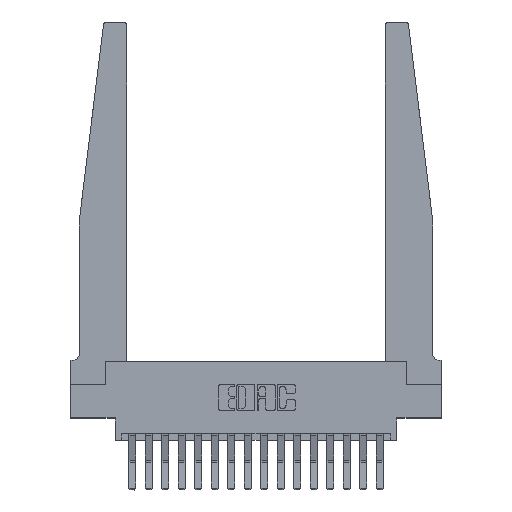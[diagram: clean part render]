
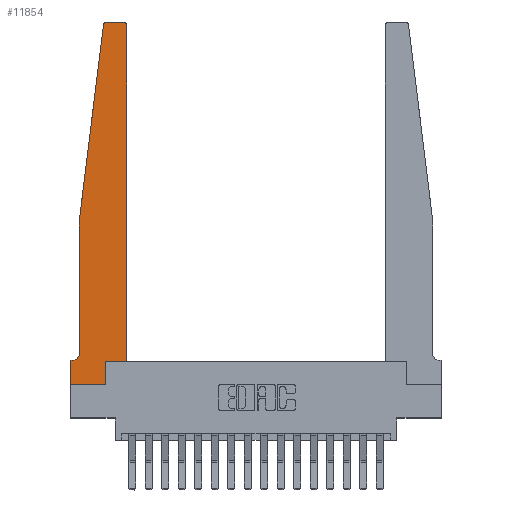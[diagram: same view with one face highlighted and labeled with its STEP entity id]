
A CAD part, top view. The second image highlights one B-rep face of the part: STEP entity #11854.
In plain terms, the highlighted planar face has unit normal (0, 0, 1).
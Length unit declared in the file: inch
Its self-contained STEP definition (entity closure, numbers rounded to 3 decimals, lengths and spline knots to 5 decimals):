
#161 = LINE ( 'NONE', #13984, #15330 ) ;
#328 = DIRECTION ( 'NONE',  ( 1., 0., 0. ) ) ;
#408 = LINE ( 'NONE', #9254, #11677 ) ;
#550 = EDGE_CURVE ( 'NONE', #15427, #4599, #3667, .T. ) ;
#650 = VERTEX_POINT ( 'NONE', #6607 ) ;
#772 = EDGE_CURVE ( 'NONE', #4599, #8223, #408, .T. ) ;
#826 = CARTESIAN_POINT ( 'NONE',  ( 0., 0., 0.37 ) ) ;
#884 = LINE ( 'NONE', #16039, #11665 ) ;
#1208 = DIRECTION ( 'NONE',  ( -1., 0., 0. ) ) ;
#1330 = EDGE_CURVE ( 'NONE', #14689, #12836, #15918, .T. ) ;
#1644 = CARTESIAN_POINT ( 'NONE',  ( 0.2605, 0.18, 0.37 ) ) ;
#1951 = CARTESIAN_POINT ( 'NONE',  ( 0.425, 0.18, 0.37 ) ) ;
#2693 = DIRECTION ( 'NONE',  ( 1., 0., 0. ) ) ;
#2923 = LINE ( 'NONE', #10007, #7752 ) ;
#3080 = EDGE_CURVE ( 'NONE', #8223, #14689, #9903, .T. ) ;
#3102 = ORIENTED_EDGE ( 'NONE', *, *, #15533, .T. ) ;
#3667 = LINE ( 'NONE', #1644, #18259 ) ;
#4114 = CARTESIAN_POINT ( 'NONE',  ( 0.065, 1.25, 0.37 ) ) ;
#4512 = CARTESIAN_POINT ( 'NONE',  ( 0.065, 1.25, 0.37 ) ) ;
#4599 = VERTEX_POINT ( 'NONE', #17142 ) ;
#4915 = CARTESIAN_POINT ( 'NONE',  ( 0.24675, 2.72367, 0.37 ) ) ;
#4948 = ORIENTED_EDGE ( 'NONE', *, *, #772, .T. ) ;
#5209 = LINE ( 'NONE', #4114, #16423 ) ;
#5229 = VERTEX_POINT ( 'NONE', #6952 ) ;
#5398 = DIRECTION ( 'NONE',  ( 1., 0., 0. ) ) ;
#5620 = AXIS2_PLACEMENT_3D ( 'NONE', #13778, #14195, #5398 ) ;
#6065 = VERTEX_POINT ( 'NONE', #4915 ) ;
#6173 = CARTESIAN_POINT ( 'NONE',  ( 0., 0.1875, 0.37 ) ) ;
#6362 = DIRECTION ( 'NONE',  ( 1., 0., 0. ) ) ;
#6607 = CARTESIAN_POINT ( 'NONE',  ( 0., 0., 0.37 ) ) ;
#6695 = DIRECTION ( 'NONE',  ( 0., 0., 1. ) ) ;
#6783 = CARTESIAN_POINT ( 'NONE',  ( 0.2605, 0., 0.37 ) ) ;
#6952 = CARTESIAN_POINT ( 'NONE',  ( 0.065, 0.2375, 0.37 ) ) ;
#6987 = ORIENTED_EDGE ( 'NONE', *, *, #18313, .T. ) ;
#7056 = EDGE_CURVE ( 'NONE', #6065, #14808, #5209, .T. ) ;
#7081 = ORIENTED_EDGE ( 'NONE', *, *, #16003, .T. ) ;
#7326 = ORIENTED_EDGE ( 'NONE', *, *, #16267, .T. ) ;
#7691 = EDGE_CURVE ( 'NONE', #5229, #14095, #18127, .T. ) ;
#7752 = VECTOR ( 'NONE', #2693, 39.37008 ) ;
#7867 = AXIS2_PLACEMENT_3D ( 'NONE', #6173, #9123, #328 ) ;
#8022 = CARTESIAN_POINT ( 'NONE',  ( 0., 0.1875, 0.37 ) ) ;
#8126 = DIRECTION ( 'NONE',  ( -1., 0., 0. ) ) ;
#8223 = VERTEX_POINT ( 'NONE', #11367 ) ;
#8530 = CARTESIAN_POINT ( 'NONE',  ( 0.425, 2.72, 0.37 ) ) ;
#8610 = CARTESIAN_POINT ( 'NONE',  ( 0.015, 0.1875, 0.37 ) ) ;
#8827 = LINE ( 'NONE', #16361, #16142 ) ;
#9123 = DIRECTION ( 'NONE',  ( 0., 0., 1. ) ) ;
#9254 = CARTESIAN_POINT ( 'NONE',  ( 0.425, 0.18, 0.37 ) ) ;
#9393 = EDGE_LOOP ( 'NONE', ( #6987, #13072, #17769, #7326, #16067, #7081, #18569, #3102, #11062, #4948, #10087, #15693 ) ) ;
#9716 = VERTEX_POINT ( 'NONE', #12044 ) ;
#9903 = LINE ( 'NONE', #1951, #17195 ) ;
#9977 = DIRECTION ( 'NONE',  ( 0., 0., -1. ) ) ;
#10007 = CARTESIAN_POINT ( 'NONE',  ( 0., 0., 0.37 ) ) ;
#10087 = ORIENTED_EDGE ( 'NONE', *, *, #3080, .T. ) ;
#10558 = DIRECTION ( 'NONE',  ( -1., 0., 0. ) ) ;
#11062 = ORIENTED_EDGE ( 'NONE', *, *, #550, .T. ) ;
#11078 = DIRECTION ( 'NONE',  ( 0., -1., 0. ) ) ;
#11193 = FACE_OUTER_BOUND ( 'NONE', #9393, .T. ) ;
#11268 = AXIS2_PLACEMENT_3D ( 'NONE', #18659, #9977, #1208 ) ;
#11367 = CARTESIAN_POINT ( 'NONE',  ( 0.425, 0.18, 0.37 ) ) ;
#11399 = EDGE_CURVE ( 'NONE', #18542, #650, #18460, .T. ) ;
#11648 = DIRECTION ( 'NONE',  ( 0., -1., 0. ) ) ;
#11665 = VECTOR ( 'NONE', #11648, 39.37008 ) ;
#11677 = VECTOR ( 'NONE', #6362, 39.37008 ) ;
#11854 = ADVANCED_FACE ( 'NONE', ( #11193 ), #16417, .T. ) ;
#12044 = CARTESIAN_POINT ( 'NONE',  ( 0.27653, 2.75, 0.37 ) ) ;
#12359 = AXIS2_PLACEMENT_3D ( 'NONE', #15479, #6695, #16927 ) ;
#12548 = DIRECTION ( 'NONE',  ( 0., 1., 0. ) ) ;
#12836 = VERTEX_POINT ( 'NONE', #14336 ) ;
#12902 = DIRECTION ( 'NONE',  ( -0.122, -0.992, 0. ) ) ;
#13072 = ORIENTED_EDGE ( 'NONE', *, *, #16009, .T. ) ;
#13778 = CARTESIAN_POINT ( 'NONE',  ( 0.395, 2.72, 0.37 ) ) ;
#13984 = CARTESIAN_POINT ( 'NONE',  ( 0.065, 0.1875, 0.37 ) ) ;
#14095 = VERTEX_POINT ( 'NONE', #8610 ) ;
#14195 = DIRECTION ( 'NONE',  ( 0., 0., 1. ) ) ;
#14205 = VECTOR ( 'NONE', #11078, 39.37008 ) ;
#14336 = CARTESIAN_POINT ( 'NONE',  ( 0.395, 2.75, 0.37 ) ) ;
#14689 = VERTEX_POINT ( 'NONE', #8530 ) ;
#14808 = VERTEX_POINT ( 'NONE', #4512 ) ;
#15330 = VECTOR ( 'NONE', #8126, 39.37008 ) ;
#15427 = VERTEX_POINT ( 'NONE', #6783 ) ;
#15479 = CARTESIAN_POINT ( 'NONE',  ( 0.27653, 2.72, 0.37 ) ) ;
#15533 = EDGE_CURVE ( 'NONE', #650, #15427, #2923, .T. ) ;
#15693 = ORIENTED_EDGE ( 'NONE', *, *, #1330, .T. ) ;
#15774 = CIRCLE ( 'NONE', #12359, 0.03 ) ;
#15918 = CIRCLE ( 'NONE', #5620, 0.03 ) ;
#16003 = EDGE_CURVE ( 'NONE', #14095, #18542, #161, .T. ) ;
#16009 = EDGE_CURVE ( 'NONE', #9716, #6065, #15774, .T. ) ;
#16039 = CARTESIAN_POINT ( 'NONE',  ( 0.065, 1.25, 0.37 ) ) ;
#16067 = ORIENTED_EDGE ( 'NONE', *, *, #7691, .T. ) ;
#16142 = VECTOR ( 'NONE', #10558, 39.37008 ) ;
#16267 = EDGE_CURVE ( 'NONE', #14808, #5229, #884, .T. ) ;
#16361 = CARTESIAN_POINT ( 'NONE',  ( 0.25, 2.75, 0.37 ) ) ;
#16417 = PLANE ( 'NONE',  #7867 ) ;
#16423 = VECTOR ( 'NONE', #12902, 39.37008 ) ;
#16534 = DIRECTION ( 'NONE',  ( 0., 1., 0. ) ) ;
#16927 = DIRECTION ( 'NONE',  ( 1., 0., 0. ) ) ;
#17142 = CARTESIAN_POINT ( 'NONE',  ( 0.2605, 0.18, 0.37 ) ) ;
#17195 = VECTOR ( 'NONE', #16534, 39.37008 ) ;
#17769 = ORIENTED_EDGE ( 'NONE', *, *, #7056, .T. ) ;
#18127 = CIRCLE ( 'NONE', #11268, 0.05 ) ;
#18259 = VECTOR ( 'NONE', #12548, 39.37008 ) ;
#18313 = EDGE_CURVE ( 'NONE', #12836, #9716, #8827, .T. ) ;
#18460 = LINE ( 'NONE', #826, #14205 ) ;
#18542 = VERTEX_POINT ( 'NONE', #8022 ) ;
#18569 = ORIENTED_EDGE ( 'NONE', *, *, #11399, .T. ) ;
#18659 = CARTESIAN_POINT ( 'NONE',  ( 0.015, 0.2375, 0.37 ) ) ;
